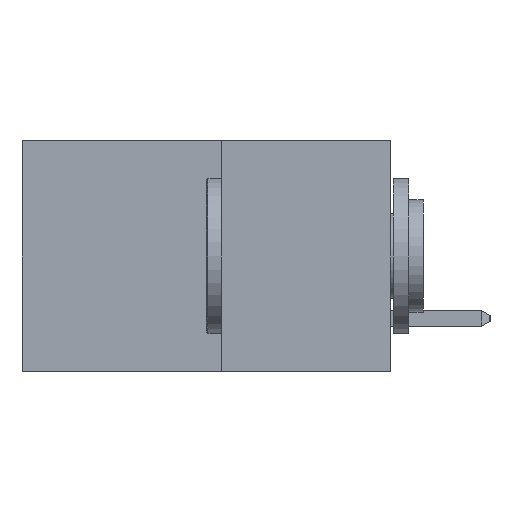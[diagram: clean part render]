
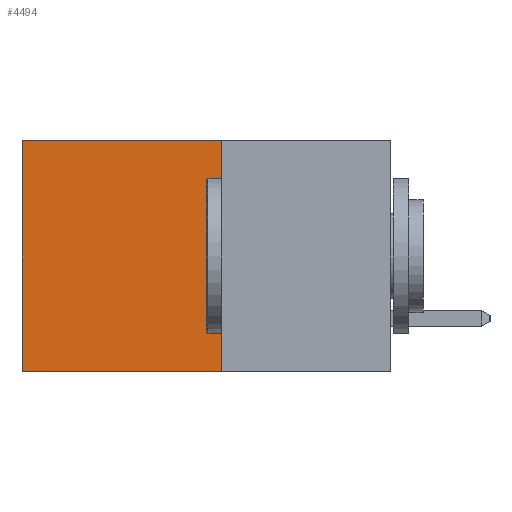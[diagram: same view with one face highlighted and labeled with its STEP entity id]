
A CAD part, left-side view. The second image highlights one B-rep face of the part: STEP entity #4494.
In plain terms, the highlighted planar face has unit normal (-1, 0, 0).
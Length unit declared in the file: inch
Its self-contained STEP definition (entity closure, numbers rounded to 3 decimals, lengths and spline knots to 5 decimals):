
#2352 = VECTOR ( 'NONE', #3846, 39.37008 ) ;
#2499 = EDGE_CURVE ( 'NONE', #9442, #2781, #4789, .T. ) ;
#2781 = VERTEX_POINT ( 'NONE', #12329 ) ;
#3077 = ORIENTED_EDGE ( 'NONE', *, *, #6028, .T. ) ;
#3209 = LINE ( 'NONE', #7900, #11041 ) ;
#3846 = DIRECTION ( 'NONE',  ( 0., 1., 0. ) ) ;
#4189 = LINE ( 'NONE', #5531, #12262 ) ;
#4334 = CARTESIAN_POINT ( 'NONE',  ( 0.277, 0.59, -0.37 ) ) ;
#4494 = ADVANCED_FACE ( 'NONE', ( #8276 ), #12115, .F. ) ;
#4562 = DIRECTION ( 'NONE',  ( 0., 0., -1. ) ) ;
#4710 = DIRECTION ( 'NONE',  ( 1., 0., 0. ) ) ;
#4789 = LINE ( 'NONE', #12153, #2352 ) ;
#4871 = ORIENTED_EDGE ( 'NONE', *, *, #10202, .F. ) ;
#5531 = CARTESIAN_POINT ( 'NONE',  ( 0.277, 0.27, -0.37 ) ) ;
#6028 = EDGE_CURVE ( 'NONE', #11100, #7521, #3209, .T. ) ;
#6060 = EDGE_LOOP ( 'NONE', ( #9630, #9014, #4871, #3077 ) ) ;
#6415 = DIRECTION ( 'NONE',  ( 0., 0., -1. ) ) ;
#7370 = LINE ( 'NONE', #4334, #9708 ) ;
#7521 = VERTEX_POINT ( 'NONE', #13171 ) ;
#7900 = CARTESIAN_POINT ( 'NONE',  ( 0.277, 0.27, 0. ) ) ;
#8199 = AXIS2_PLACEMENT_3D ( 'NONE', #12848, #4710, #4562 ) ;
#8276 = FACE_OUTER_BOUND ( 'NONE', #6060, .T. ) ;
#9014 = ORIENTED_EDGE ( 'NONE', *, *, #2499, .F. ) ;
#9442 = VERTEX_POINT ( 'NONE', #11031 ) ;
#9630 = ORIENTED_EDGE ( 'NONE', *, *, #12108, .T. ) ;
#9708 = VECTOR ( 'NONE', #6415, 39.37008 ) ;
#9832 = CARTESIAN_POINT ( 'NONE',  ( 0.277, 0.27, 0. ) ) ;
#10202 = EDGE_CURVE ( 'NONE', #11100, #9442, #4189, .T. ) ;
#10923 = DIRECTION ( 'NONE',  ( 0., 1., 0. ) ) ;
#11031 = CARTESIAN_POINT ( 'NONE',  ( 0.277, 0.27, -0.37 ) ) ;
#11041 = VECTOR ( 'NONE', #10923, 39.37008 ) ;
#11100 = VERTEX_POINT ( 'NONE', #9832 ) ;
#12108 = EDGE_CURVE ( 'NONE', #7521, #2781, #7370, .T. ) ;
#12115 = PLANE ( 'NONE',  #8199 ) ;
#12153 = CARTESIAN_POINT ( 'NONE',  ( 0.277, 0.27, -0.37 ) ) ;
#12262 = VECTOR ( 'NONE', #12555, 39.37008 ) ;
#12329 = CARTESIAN_POINT ( 'NONE',  ( 0.277, 0.59, -0.37 ) ) ;
#12555 = DIRECTION ( 'NONE',  ( 0., 0., -1. ) ) ;
#12848 = CARTESIAN_POINT ( 'NONE',  ( 0.277, 0.27, -0.37 ) ) ;
#13171 = CARTESIAN_POINT ( 'NONE',  ( 0.277, 0.59, 0. ) ) ;
